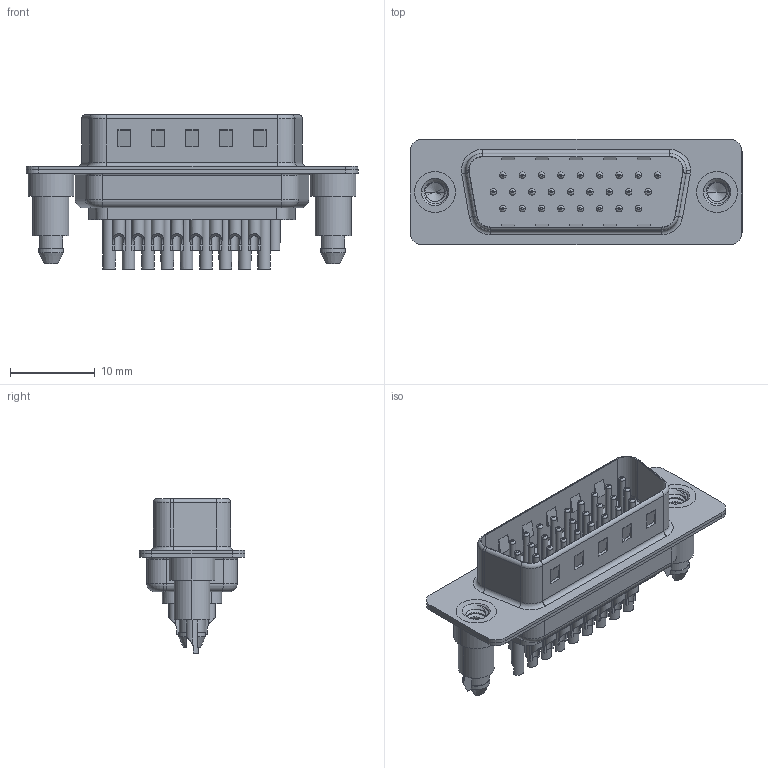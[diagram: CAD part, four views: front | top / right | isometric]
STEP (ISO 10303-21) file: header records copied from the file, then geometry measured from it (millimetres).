
FILE_DESCRIPTION (( 'STEP AP203' ), '1' );
FILE_NAME ('637-M26-332-BN5.STEP', '2018-11-19T23:53:01', ( '' ), ( '' ), 'SwSTEP 2.0', 'SolidWorks 2016', '' );
FILE_SCHEMA (( 'CONFIG_CONTROL_DESIGN' ));
Length unit declared in the file: millimetre
Products named in the file (8): 637M 4-40 Threaded Boardlock; 637-M26-332-BN5; 637M Housing_26 Contacts; 637M Shell Front_26 Contacts; 637M Shell Rear_26 Contacts; 637M Contact Row 1_32; 637M Contact Row 2_32; 637M Contact Row 3_32
Assembly tree (31 placements, depth 2):
  637-M26-332-BN5
    637M Housing_26 Contacts
    637M Shell Front_26 Contacts
    637M Shell Rear_26 Contacts
    637M Contact Row 1_32  x9
    637M Contact Row 2_32  x9
    637M Contact Row 3_32  x8
    637M 4-40 Threaded Boardlock  x2
Bounding box: 39.2 x 12.5 x 18.25 mm (x, y, z)
Volume: 2129.4 mm3; surface area: 6406.3 mm2
Topology: 31 solids, 31 shells, 1352 faces, 3173 edges, 1950 vertices
Faces by surface type: cylinder 581, plane 389, torus 310, cone 66, bspline 6
Entity records: 21732 total; most frequent: CARTESIAN_POINT 5001, DIRECTION 3419, ORIENTED_EDGE 3000, EDGE_CURVE 1500, AXIS2_PLACEMENT_3D 1363, VERTEX_POINT 958, EDGE_LOOP 782, CIRCLE 705
